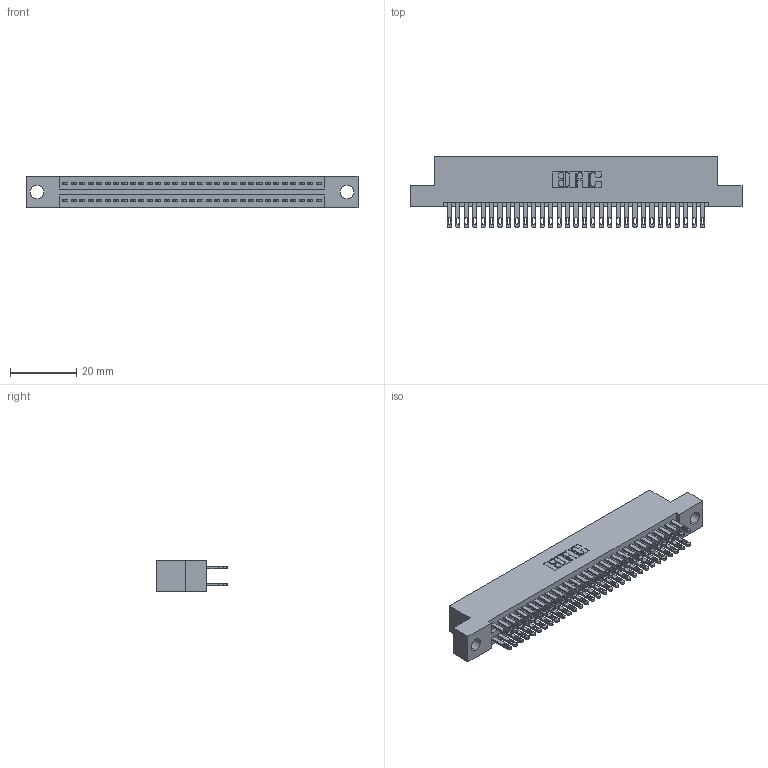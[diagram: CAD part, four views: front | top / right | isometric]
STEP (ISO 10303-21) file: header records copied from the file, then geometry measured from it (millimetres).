
FILE_DESCRIPTION (( 'STEP AP203' ), '1' );
FILE_NAME ('895-062-500-204.STEP', '2020-09-28T07:03:30', ( '' ), ( '' ), 'SwSTEP 2.0', 'SolidWorks 2020', '' );
FILE_SCHEMA (( 'CONFIG_CONTROL_DESIGN' ));
Length unit declared in the file: inch
Products named in the file (3): 345-292-001_345-293-100; 895-062-500-204; 845 Part_Flush Mounting Lugs - 0.156 Dia-TH
Assembly tree (63 placements, depth 2):
  895-062-500-204
    845 Part_Flush Mounting Lugs - 0.156 Dia-TH
    345-292-001_345-293-100  x62
Bounding box: 99.95 x 21.51 x 9.4 mm (x, y, z)
Volume: 9708.6 mm3; surface area: 14585.5 mm2
Topology: 63 solids, 63 shells, 2978 faces, 9083 edges, 6054 vertices
Faces by surface type: plane 1754, cylinder 1224
Entity records: 25737 total; most frequent: CARTESIAN_POINT 4324, ORIENTED_EDGE 4258, DIRECTION 3829, EDGE_CURVE 2129, VECTOR 1869, LINE 1869, VERTEX_POINT 1418, AXIS2_PLACEMENT_3D 980
